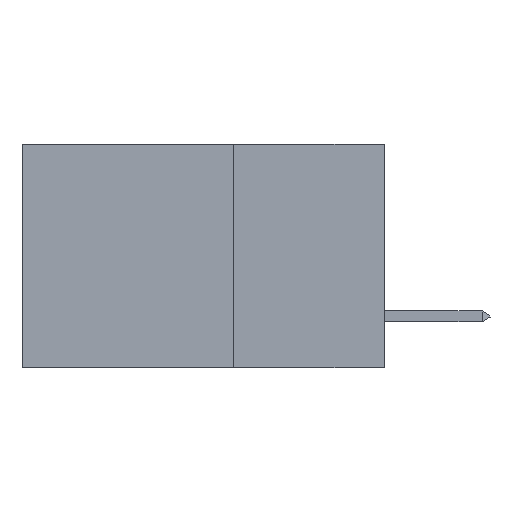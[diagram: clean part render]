
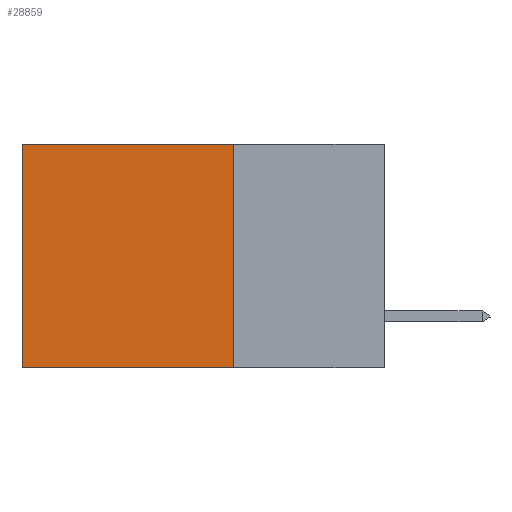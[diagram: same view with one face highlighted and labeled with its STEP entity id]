
A CAD part, left-side view. The second image highlights one B-rep face of the part: STEP entity #28859.
In plain terms, the highlighted planar face has unit normal (-1, 0, 0).
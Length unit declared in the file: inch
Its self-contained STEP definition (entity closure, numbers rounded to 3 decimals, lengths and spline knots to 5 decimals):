
#1510 = LINE ( 'NONE', #12461, #2111 ) ;
#1620 = VECTOR ( 'NONE', #17222, 39.37008 ) ;
#2111 = VECTOR ( 'NONE', #45621, 39.37008 ) ;
#3568 = LINE ( 'NONE', #6991, #43306 ) ;
#4906 = DIRECTION ( 'NONE',  ( 0., 0., -1. ) ) ;
#5225 = CARTESIAN_POINT ( 'NONE',  ( 0.2875, 0.25, 0. ) ) ;
#6876 = EDGE_CURVE ( 'NONE', #35631, #30456, #23551, .T. ) ;
#6991 = CARTESIAN_POINT ( 'NONE',  ( 0.2875, 0.25, -0.37 ) ) ;
#7260 = CARTESIAN_POINT ( 'NONE',  ( 0.2875, 0.25, -0.37 ) ) ;
#8818 = VERTEX_POINT ( 'NONE', #41035 ) ;
#12461 = CARTESIAN_POINT ( 'NONE',  ( 0.2875, 0.25, 0. ) ) ;
#12723 = EDGE_CURVE ( 'NONE', #13103, #8818, #26149, .T. ) ;
#13103 = VERTEX_POINT ( 'NONE', #36166 ) ;
#17222 = DIRECTION ( 'NONE',  ( 0., 0., -1. ) ) ;
#20870 = ORIENTED_EDGE ( 'NONE', *, *, #6876, .F. ) ;
#20988 = CARTESIAN_POINT ( 'NONE',  ( 0.2875, 0.6, 0. ) ) ;
#23551 = LINE ( 'NONE', #24306, #1620 ) ;
#24306 = CARTESIAN_POINT ( 'NONE',  ( 0.2875, 0.25, 0. ) ) ;
#26149 = LINE ( 'NONE', #20988, #40526 ) ;
#28619 = EDGE_CURVE ( 'NONE', #30456, #8818, #3568, .T. ) ;
#28859 = ADVANCED_FACE ( 'NONE', ( #28905 ), #41906, .F. ) ;
#28905 = FACE_OUTER_BOUND ( 'NONE', #32339, .T. ) ;
#29068 = DIRECTION ( 'NONE',  ( 0., 1., 0. ) ) ;
#30456 = VERTEX_POINT ( 'NONE', #7260 ) ;
#30894 = ORIENTED_EDGE ( 'NONE', *, *, #33451, .T. ) ;
#32339 = EDGE_LOOP ( 'NONE', ( #43967, #40785, #20870, #30894 ) ) ;
#33451 = EDGE_CURVE ( 'NONE', #35631, #13103, #1510, .T. ) ;
#35631 = VERTEX_POINT ( 'NONE', #38592 ) ;
#36166 = CARTESIAN_POINT ( 'NONE',  ( 0.2875, 0.6, 0. ) ) ;
#37938 = AXIS2_PLACEMENT_3D ( 'NONE', #5225, #41584, #4906 ) ;
#38592 = CARTESIAN_POINT ( 'NONE',  ( 0.2875, 0.25, 0. ) ) ;
#40526 = VECTOR ( 'NONE', #46702, 39.37008 ) ;
#40785 = ORIENTED_EDGE ( 'NONE', *, *, #28619, .F. ) ;
#41035 = CARTESIAN_POINT ( 'NONE',  ( 0.2875, 0.6, -0.37 ) ) ;
#41584 = DIRECTION ( 'NONE',  ( 1., 0., 0. ) ) ;
#41906 = PLANE ( 'NONE',  #37938 ) ;
#43306 = VECTOR ( 'NONE', #29068, 39.37008 ) ;
#43967 = ORIENTED_EDGE ( 'NONE', *, *, #12723, .T. ) ;
#45621 = DIRECTION ( 'NONE',  ( 0., 1., 0. ) ) ;
#46702 = DIRECTION ( 'NONE',  ( 0., 0., -1. ) ) ;
